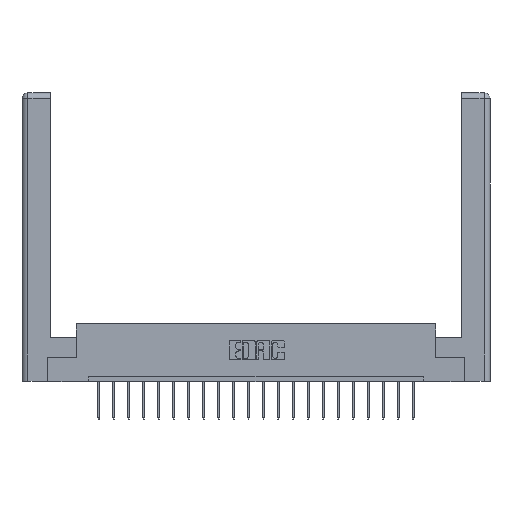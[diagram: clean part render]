
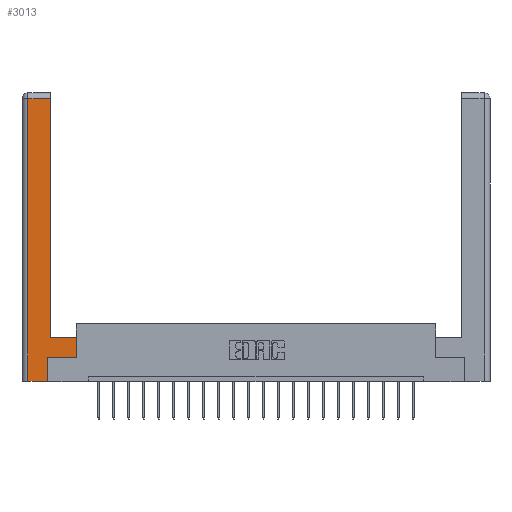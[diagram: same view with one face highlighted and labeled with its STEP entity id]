
A CAD part, top view. The second image highlights one B-rep face of the part: STEP entity #3013.
In plain terms, the highlighted planar face has unit normal (0, 0, 1).
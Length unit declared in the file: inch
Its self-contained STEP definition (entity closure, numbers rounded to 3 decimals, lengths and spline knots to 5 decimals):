
#909 = CARTESIAN_POINT ( 'NONE',  ( 0.265, 0.245, 0. ) ) ;
#1100 = LINE ( 'NONE', #19349, #2153 ) ;
#2042 = DIRECTION ( 'NONE',  ( 1., 0., 0. ) ) ;
#2050 = LINE ( 'NONE', #18994, #12203 ) ;
#2153 = VECTOR ( 'NONE', #17871, 39.37008 ) ;
#2171 = EDGE_CURVE ( 'NONE', #5681, #16768, #10573, .T. ) ;
#2409 = VECTOR ( 'NONE', #16284, 39.37008 ) ;
#2951 = PLANE ( 'NONE',  #11743 ) ;
#3013 = ADVANCED_FACE ( 'NONE', ( #3415 ), #2951, .F. ) ;
#3110 = CARTESIAN_POINT ( 'NONE',  ( 0.0615, 0., 0. ) ) ;
#3397 = CARTESIAN_POINT ( 'NONE',  ( 0.295, 0.45, 0. ) ) ;
#3415 = FACE_OUTER_BOUND ( 'NONE', #6809, .T. ) ;
#4616 = CARTESIAN_POINT ( 'NONE',  ( 0., 0., 0. ) ) ;
#4750 = CARTESIAN_POINT ( 'NONE',  ( 0.565, 0.245, 0. ) ) ;
#5681 = VERTEX_POINT ( 'NONE', #3110 ) ;
#5777 = VERTEX_POINT ( 'NONE', #16956 ) ;
#6809 = EDGE_LOOP ( 'NONE', ( #9755, #8902, #9487, #12042, #14936, #9635, #7457, #13390 ) ) ;
#7275 = VERTEX_POINT ( 'NONE', #14850 ) ;
#7457 = ORIENTED_EDGE ( 'NONE', *, *, #16844, .T. ) ;
#8064 = CARTESIAN_POINT ( 'NONE',  ( 0.0615, 0., 0. ) ) ;
#8506 = LINE ( 'NONE', #10737, #12135 ) ;
#8902 = ORIENTED_EDGE ( 'NONE', *, *, #12034, .T. ) ;
#8953 = CARTESIAN_POINT ( 'NONE',  ( 0.265, 0., 0. ) ) ;
#9089 = EDGE_CURVE ( 'NONE', #14693, #13876, #10023, .T. ) ;
#9487 = ORIENTED_EDGE ( 'NONE', *, *, #20106, .T. ) ;
#9635 = ORIENTED_EDGE ( 'NONE', *, *, #9089, .T. ) ;
#9755 = ORIENTED_EDGE ( 'NONE', *, *, #13304, .T. ) ;
#10023 = LINE ( 'NONE', #21292, #18679 ) ;
#10300 = CARTESIAN_POINT ( 'NONE',  ( 0.0615, 2.94, 0. ) ) ;
#10412 = CARTESIAN_POINT ( 'NONE',  ( 0.0615, 2.94, 0. ) ) ;
#10573 = LINE ( 'NONE', #11647, #16061 ) ;
#10737 = CARTESIAN_POINT ( 'NONE',  ( 0.295, 0.45, 0. ) ) ;
#10828 = EDGE_CURVE ( 'NONE', #16768, #14693, #1100, .T. ) ;
#11647 = CARTESIAN_POINT ( 'NONE',  ( 0.265, 0., 0. ) ) ;
#11743 = AXIS2_PLACEMENT_3D ( 'NONE', #4616, #16343, #14747 ) ;
#12034 = EDGE_CURVE ( 'NONE', #5777, #20918, #16734, .T. ) ;
#12042 = ORIENTED_EDGE ( 'NONE', *, *, #2171, .T. ) ;
#12135 = VECTOR ( 'NONE', #17186, 39.37008 ) ;
#12203 = VECTOR ( 'NONE', #14005, 39.37008 ) ;
#13304 = EDGE_CURVE ( 'NONE', #15240, #5777, #2050, .T. ) ;
#13390 = ORIENTED_EDGE ( 'NONE', *, *, #14597, .T. ) ;
#13876 = VERTEX_POINT ( 'NONE', #4750 ) ;
#14005 = DIRECTION ( 'NONE',  ( 0., 1., 0. ) ) ;
#14296 = DIRECTION ( 'NONE',  ( 0., 1., 0. ) ) ;
#14597 = EDGE_CURVE ( 'NONE', #7275, #15240, #8506, .T. ) ;
#14693 = VERTEX_POINT ( 'NONE', #909 ) ;
#14747 = DIRECTION ( 'NONE',  ( -1., 0., 0. ) ) ;
#14850 = CARTESIAN_POINT ( 'NONE',  ( 0.565, 0.45, 0. ) ) ;
#14936 = ORIENTED_EDGE ( 'NONE', *, *, #10828, .T. ) ;
#15070 = VECTOR ( 'NONE', #14296, 39.37008 ) ;
#15240 = VERTEX_POINT ( 'NONE', #3397 ) ;
#15316 = LINE ( 'NONE', #17440, #15070 ) ;
#16061 = VECTOR ( 'NONE', #2042, 39.37008 ) ;
#16284 = DIRECTION ( 'NONE',  ( 0., -1., 0. ) ) ;
#16343 = DIRECTION ( 'NONE',  ( 0., 0., -1. ) ) ;
#16462 = VECTOR ( 'NONE', #18818, 39.37008 ) ;
#16734 = LINE ( 'NONE', #10300, #16462 ) ;
#16768 = VERTEX_POINT ( 'NONE', #8953 ) ;
#16844 = EDGE_CURVE ( 'NONE', #13876, #7275, #15316, .T. ) ;
#16956 = CARTESIAN_POINT ( 'NONE',  ( 0.295, 2.94, 0. ) ) ;
#17186 = DIRECTION ( 'NONE',  ( -1., 0., 0. ) ) ;
#17440 = CARTESIAN_POINT ( 'NONE',  ( 0.565, 0.45, 0. ) ) ;
#17656 = DIRECTION ( 'NONE',  ( 1., 0., 0. ) ) ;
#17871 = DIRECTION ( 'NONE',  ( 0., 1., 0. ) ) ;
#18679 = VECTOR ( 'NONE', #17656, 39.37008 ) ;
#18818 = DIRECTION ( 'NONE',  ( -1., 0., 0. ) ) ;
#18994 = CARTESIAN_POINT ( 'NONE',  ( 0.295, 3., 0. ) ) ;
#19349 = CARTESIAN_POINT ( 'NONE',  ( 0.265, 0.245, 0. ) ) ;
#20106 = EDGE_CURVE ( 'NONE', #20918, #5681, #20919, .T. ) ;
#20918 = VERTEX_POINT ( 'NONE', #10412 ) ;
#20919 = LINE ( 'NONE', #8064, #2409 ) ;
#21292 = CARTESIAN_POINT ( 'NONE',  ( 0.565, 0.245, 0. ) ) ;
